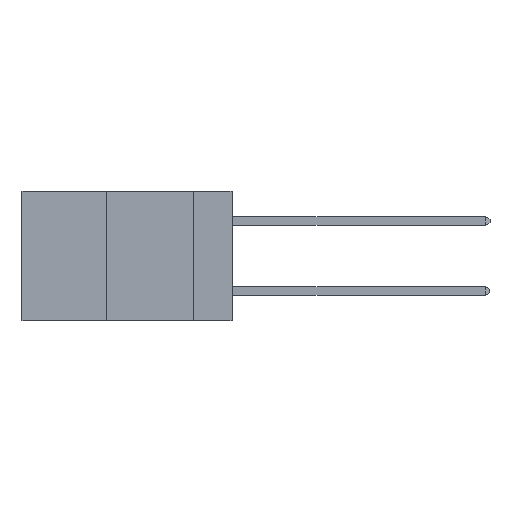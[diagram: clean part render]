
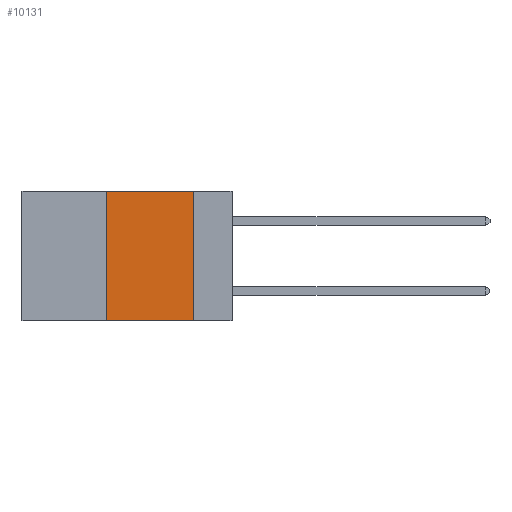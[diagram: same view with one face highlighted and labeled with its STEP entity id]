
A CAD part, left-side view. The second image highlights one B-rep face of the part: STEP entity #10131.
In plain terms, the highlighted planar face has unit normal (-1, 0, 0).
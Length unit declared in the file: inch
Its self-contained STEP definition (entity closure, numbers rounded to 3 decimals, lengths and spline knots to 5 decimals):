
#41 = VERTEX_POINT ( 'NONE', #4759 ) ;
#83 = VERTEX_POINT ( 'NONE', #1360 ) ;
#154 = DIRECTION ( 'NONE',  ( 0., -1., 0. ) ) ;
#360 = EDGE_LOOP ( 'NONE', ( #5564, #10235, #5818, #8203 ) ) ;
#835 = LINE ( 'NONE', #8185, #3415 ) ;
#1017 = AXIS2_PLACEMENT_3D ( 'NONE', #10835, #11633, #6481 ) ;
#1360 = CARTESIAN_POINT ( 'NONE',  ( 0., 0.36, -0.37 ) ) ;
#2356 = CARTESIAN_POINT ( 'NONE',  ( 0., 0.36, 0. ) ) ;
#2530 = VERTEX_POINT ( 'NONE', #5388 ) ;
#3415 = VECTOR ( 'NONE', #7252, 39.37008 ) ;
#4638 = EDGE_CURVE ( 'NONE', #83, #8743, #11099, .T. ) ;
#4750 = PLANE ( 'NONE',  #1017 ) ;
#4759 = CARTESIAN_POINT ( 'NONE',  ( 0., 0.11, -0.37 ) ) ;
#4777 = CARTESIAN_POINT ( 'NONE',  ( 0., 0.36, 0. ) ) ;
#4965 = EDGE_CURVE ( 'NONE', #8743, #2530, #835, .T. ) ;
#5010 = DIRECTION ( 'NONE',  ( 0., 0., -1. ) ) ;
#5115 = DIRECTION ( 'NONE',  ( 0., 0., 1. ) ) ;
#5246 = EDGE_CURVE ( 'NONE', #2530, #41, #5405, .T. ) ;
#5388 = CARTESIAN_POINT ( 'NONE',  ( 0., 0.11, 0. ) ) ;
#5405 = LINE ( 'NONE', #10260, #9816 ) ;
#5564 = ORIENTED_EDGE ( 'NONE', *, *, #5246, .F. ) ;
#5818 = ORIENTED_EDGE ( 'NONE', *, *, #4638, .F. ) ;
#6481 = DIRECTION ( 'NONE',  ( 0., 0., -1. ) ) ;
#6925 = LINE ( 'NONE', #9389, #9060 ) ;
#7252 = DIRECTION ( 'NONE',  ( 0., -1., 0. ) ) ;
#7421 = EDGE_CURVE ( 'NONE', #83, #41, #6925, .T. ) ;
#8185 = CARTESIAN_POINT ( 'NONE',  ( 0., 0.6, 0. ) ) ;
#8203 = ORIENTED_EDGE ( 'NONE', *, *, #7421, .T. ) ;
#8595 = VECTOR ( 'NONE', #5115, 39.37008 ) ;
#8743 = VERTEX_POINT ( 'NONE', #4777 ) ;
#9060 = VECTOR ( 'NONE', #154, 39.37008 ) ;
#9389 = CARTESIAN_POINT ( 'NONE',  ( 0., 0.6, -0.37 ) ) ;
#9816 = VECTOR ( 'NONE', #5010, 39.37008 ) ;
#10131 = ADVANCED_FACE ( 'NONE', ( #10962 ), #4750, .F. ) ;
#10235 = ORIENTED_EDGE ( 'NONE', *, *, #4965, .F. ) ;
#10260 = CARTESIAN_POINT ( 'NONE',  ( 0., 0.11, 0. ) ) ;
#10835 = CARTESIAN_POINT ( 'NONE',  ( 0., 0.6, 0. ) ) ;
#10962 = FACE_OUTER_BOUND ( 'NONE', #360, .T. ) ;
#11099 = LINE ( 'NONE', #2356, #8595 ) ;
#11633 = DIRECTION ( 'NONE',  ( 1., 0., 0. ) ) ;
